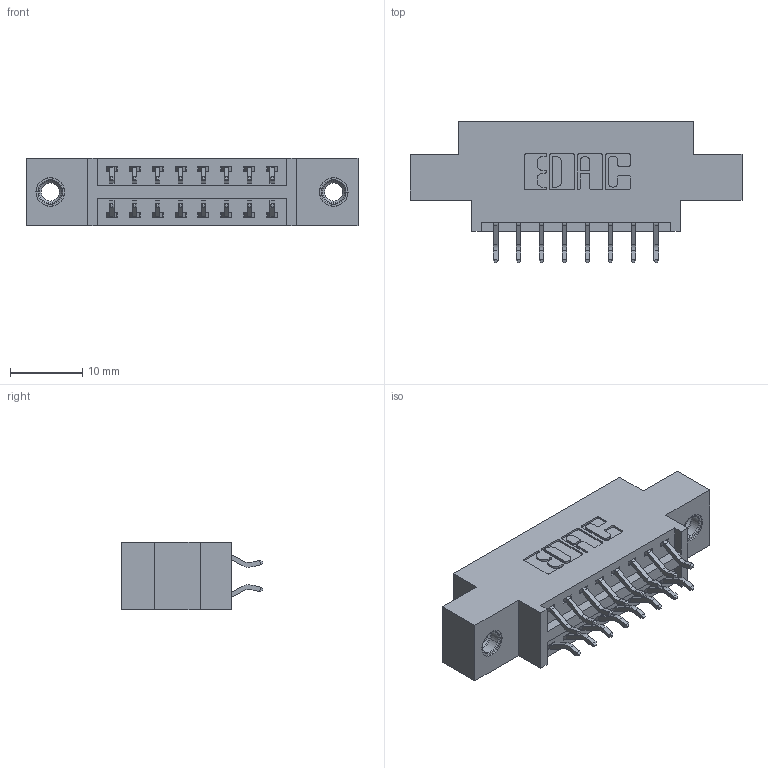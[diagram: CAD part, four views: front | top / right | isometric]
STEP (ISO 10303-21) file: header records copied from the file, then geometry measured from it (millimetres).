
FILE_DESCRIPTION (( 'STEP AP203' ), '1' );
FILE_NAME ('346-016-556-807.STEP', '2022-05-18T16:18:10', ( '' ), ( '' ), 'SwSTEP 2.0', 'SolidWorks 2020', '' );
FILE_SCHEMA (( 'CONFIG_CONTROL_DESIGN' ));
Length unit declared in the file: inch
Products named in the file (4): 346 Part_0.170 Offset - 0.156 Dia-TI; 345-292-001_556 Tail; 346-016-556-807; 345-250-001_345-250-005-103
Assembly tree (19 placements, depth 2):
  346-016-556-807
    346 Part_0.170 Offset - 0.156 Dia-TI
    345-292-001_556 Tail  x16
    345-250-001_345-250-005-103  x2
Bounding box: 45.97 x 19.57 x 9.4 mm (x, y, z)
Volume: 4050.2 mm3; surface area: 5231.4 mm2
Topology: 19 solids, 19 shells, 1114 faces, 3245 edges, 2134 vertices
Faces by surface type: plane 736, cylinder 362, cone 12, torus 4
Entity records: 11336 total; most frequent: CARTESIAN_POINT 1915, ORIENTED_EDGE 1830, DIRECTION 1753, EDGE_CURVE 915, VECTOR 723, LINE 723, VERTEX_POINT 604, AXIS2_PLACEMENT_3D 515
